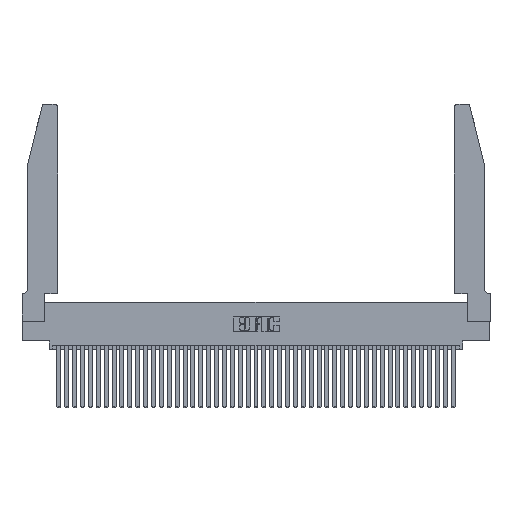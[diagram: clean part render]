
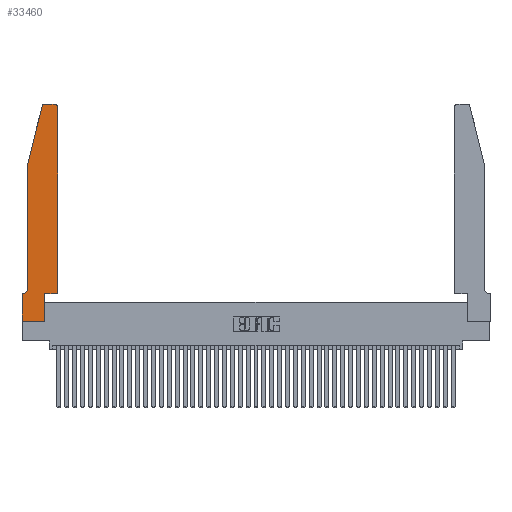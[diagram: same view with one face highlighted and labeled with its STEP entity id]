
A CAD part, top view. The second image highlights one B-rep face of the part: STEP entity #33460.
In plain terms, the highlighted planar face has unit normal (0, 0, 1).
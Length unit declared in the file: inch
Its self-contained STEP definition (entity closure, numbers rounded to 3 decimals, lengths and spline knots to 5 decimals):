
#149 = VECTOR ( 'NONE', #41170, 39.37008 ) ;
#591 = ORIENTED_EDGE ( 'NONE', *, *, #41050, .T. ) ;
#843 = CARTESIAN_POINT ( 'NONE',  ( 0.25487, 2.72718, 0.37 ) ) ;
#1195 = VECTOR ( 'NONE', #23266, 39.37008 ) ;
#1265 = LINE ( 'NONE', #6228, #8586 ) ;
#1380 = DIRECTION ( 'NONE',  ( -1., 0., 0. ) ) ;
#2826 = CARTESIAN_POINT ( 'NONE',  ( 0.0755, 0.35, 0.37 ) ) ;
#3348 = ORIENTED_EDGE ( 'NONE', *, *, #5975, .T. ) ;
#4459 = CARTESIAN_POINT ( 'NONE',  ( 0.2865, 0.35, 0.37 ) ) ;
#5761 = VERTEX_POINT ( 'NONE', #24829 ) ;
#5888 = ORIENTED_EDGE ( 'NONE', *, *, #37922, .T. ) ;
#5975 = EDGE_CURVE ( 'NONE', #10247, #7414, #9062, .T. ) ;
#6228 = CARTESIAN_POINT ( 'NONE',  ( 0., 0., 0.37 ) ) ;
#6584 = VECTOR ( 'NONE', #27744, 39.37008 ) ;
#6618 = VECTOR ( 'NONE', #22901, 39.37008 ) ;
#7010 = ORIENTED_EDGE ( 'NONE', *, *, #17214, .T. ) ;
#7385 = CARTESIAN_POINT ( 'NONE',  ( 0.284, 2.72, 0.37 ) ) ;
#7414 = VERTEX_POINT ( 'NONE', #34551 ) ;
#7542 = EDGE_CURVE ( 'NONE', #10661, #35341, #28443, .T. ) ;
#7826 = DIRECTION ( 'NONE',  ( 1., 0., 0. ) ) ;
#7898 = CARTESIAN_POINT ( 'NONE',  ( 0.4505, 0.35, 0.37 ) ) ;
#8586 = VECTOR ( 'NONE', #12844, 39.37008 ) ;
#8888 = VECTOR ( 'NONE', #24310, 39.37008 ) ;
#8977 = VECTOR ( 'NONE', #29935, 39.37008 ) ;
#9014 = VERTEX_POINT ( 'NONE', #22245 ) ;
#9062 = LINE ( 'NONE', #2826, #1195 ) ;
#9153 = CIRCLE ( 'NONE', #35508, 0.03 ) ;
#9172 = CARTESIAN_POINT ( 'NONE',  ( 0.4205, 2.75, 0.37 ) ) ;
#9303 = ORIENTED_EDGE ( 'NONE', *, *, #29310, .T. ) ;
#9967 = AXIS2_PLACEMENT_3D ( 'NONE', #7385, #27265, #30627 ) ;
#10138 = LINE ( 'NONE', #4459, #149 ) ;
#10247 = VERTEX_POINT ( 'NONE', #21009 ) ;
#10661 = VERTEX_POINT ( 'NONE', #9172 ) ;
#10894 = ORIENTED_EDGE ( 'NONE', *, *, #7542, .T. ) ;
#10961 = CARTESIAN_POINT ( 'NONE',  ( 0.0755, 2., 0.37 ) ) ;
#11203 = PLANE ( 'NONE',  #42043 ) ;
#11349 = CARTESIAN_POINT ( 'NONE',  ( 0., 0.35, 0.37 ) ) ;
#12844 = DIRECTION ( 'NONE',  ( 0., -1., 0. ) ) ;
#14658 = DIRECTION ( 'NONE',  ( 0., 0., -1. ) ) ;
#16202 = DIRECTION ( 'NONE',  ( 0., 0., 1. ) ) ;
#16878 = LINE ( 'NONE', #7898, #19493 ) ;
#17214 = EDGE_CURVE ( 'NONE', #35341, #30072, #18837, .T. ) ;
#17761 = CARTESIAN_POINT ( 'NONE',  ( 0.0755, 2., 0.37 ) ) ;
#17921 = LINE ( 'NONE', #24764, #8977 ) ;
#18352 = EDGE_CURVE ( 'NONE', #5761, #26841, #16878, .T. ) ;
#18398 = EDGE_CURVE ( 'NONE', #26841, #34080, #17921, .T. ) ;
#18837 = CIRCLE ( 'NONE', #9967, 0.03 ) ;
#19493 = VECTOR ( 'NONE', #28366, 39.37008 ) ;
#20409 = CARTESIAN_POINT ( 'NONE',  ( 0.2605, 2.75, 0.37 ) ) ;
#21009 = CARTESIAN_POINT ( 'NONE',  ( 0.0055, 0.35, 0.37 ) ) ;
#21439 = VERTEX_POINT ( 'NONE', #17761 ) ;
#21795 = CARTESIAN_POINT ( 'NONE',  ( 0.4505, 2.72, 0.37 ) ) ;
#22245 = CARTESIAN_POINT ( 'NONE',  ( 0.2865, 0., 0.37 ) ) ;
#22258 = CARTESIAN_POINT ( 'NONE',  ( 0.0755, 0.42, 0.37 ) ) ;
#22901 = DIRECTION ( 'NONE',  ( 0., -1., 0. ) ) ;
#23266 = DIRECTION ( 'NONE',  ( -1., 0., 0. ) ) ;
#23554 = VERTEX_POINT ( 'NONE', #22258 ) ;
#24310 = DIRECTION ( 'NONE',  ( 1., 0., 0. ) ) ;
#24764 = CARTESIAN_POINT ( 'NONE',  ( 0.4505, 0.35, 0.37 ) ) ;
#24829 = CARTESIAN_POINT ( 'NONE',  ( 0.2865, 0.35, 0.37 ) ) ;
#24857 = CARTESIAN_POINT ( 'NONE',  ( 0., 0., 0.37 ) ) ;
#25534 = ORIENTED_EDGE ( 'NONE', *, *, #18352, .T. ) ;
#25536 = ORIENTED_EDGE ( 'NONE', *, *, #37291, .T. ) ;
#26841 = VERTEX_POINT ( 'NONE', #43111 ) ;
#27265 = DIRECTION ( 'NONE',  ( 0., 0., 1. ) ) ;
#27547 = EDGE_CURVE ( 'NONE', #21439, #23554, #36650, .T. ) ;
#27744 = DIRECTION ( 'NONE',  ( -0.239, -0.971, 0. ) ) ;
#28271 = LINE ( 'NONE', #10961, #6584 ) ;
#28366 = DIRECTION ( 'NONE',  ( 1., 0., 0. ) ) ;
#28381 = ORIENTED_EDGE ( 'NONE', *, *, #37279, .T. ) ;
#28443 = LINE ( 'NONE', #20409, #42631 ) ;
#29310 = EDGE_CURVE ( 'NONE', #34080, #10661, #9153, .T. ) ;
#29935 = DIRECTION ( 'NONE',  ( 0., 1., 0. ) ) ;
#30072 = VERTEX_POINT ( 'NONE', #843 ) ;
#30408 = EDGE_LOOP ( 'NONE', ( #10894, #7010, #25536, #35994, #28381, #3348, #40941, #5888, #591, #25534, #38029, #9303 ) ) ;
#30627 = DIRECTION ( 'NONE',  ( 1., 0., 0. ) ) ;
#32799 = CARTESIAN_POINT ( 'NONE',  ( 0.4205, 2.72, 0.37 ) ) ;
#33460 = ADVANCED_FACE ( 'NONE', ( #33469 ), #11203, .T. ) ;
#33469 = FACE_OUTER_BOUND ( 'NONE', #30408, .T. ) ;
#34080 = VERTEX_POINT ( 'NONE', #21795 ) ;
#34312 = CARTESIAN_POINT ( 'NONE',  ( 0., 0., 0.37 ) ) ;
#34551 = CARTESIAN_POINT ( 'NONE',  ( 0., 0.35, 0.37 ) ) ;
#34752 = DIRECTION ( 'NONE',  ( 0., 0., 1. ) ) ;
#35109 = AXIS2_PLACEMENT_3D ( 'NONE', #41700, #14658, #37895 ) ;
#35142 = CARTESIAN_POINT ( 'NONE',  ( 0.0755, 2., 0.37 ) ) ;
#35341 = VERTEX_POINT ( 'NONE', #37178 ) ;
#35508 = AXIS2_PLACEMENT_3D ( 'NONE', #32799, #16202, #39472 ) ;
#35812 = EDGE_CURVE ( 'NONE', #7414, #36731, #1265, .T. ) ;
#35994 = ORIENTED_EDGE ( 'NONE', *, *, #27547, .T. ) ;
#36284 = LINE ( 'NONE', #34312, #8888 ) ;
#36650 = LINE ( 'NONE', #35142, #6618 ) ;
#36731 = VERTEX_POINT ( 'NONE', #24857 ) ;
#37178 = CARTESIAN_POINT ( 'NONE',  ( 0.284, 2.75, 0.37 ) ) ;
#37279 = EDGE_CURVE ( 'NONE', #23554, #10247, #40167, .T. ) ;
#37291 = EDGE_CURVE ( 'NONE', #30072, #21439, #28271, .T. ) ;
#37895 = DIRECTION ( 'NONE',  ( -1., 0., 0. ) ) ;
#37922 = EDGE_CURVE ( 'NONE', #36731, #9014, #36284, .T. ) ;
#38029 = ORIENTED_EDGE ( 'NONE', *, *, #18398, .T. ) ;
#39472 = DIRECTION ( 'NONE',  ( 1., 0., 0. ) ) ;
#40167 = CIRCLE ( 'NONE', #35109, 0.07 ) ;
#40941 = ORIENTED_EDGE ( 'NONE', *, *, #35812, .T. ) ;
#41050 = EDGE_CURVE ( 'NONE', #9014, #5761, #10138, .T. ) ;
#41170 = DIRECTION ( 'NONE',  ( 0., 1., 0. ) ) ;
#41700 = CARTESIAN_POINT ( 'NONE',  ( 0.0055, 0.42, 0.37 ) ) ;
#42043 = AXIS2_PLACEMENT_3D ( 'NONE', #11349, #34752, #7826 ) ;
#42631 = VECTOR ( 'NONE', #1380, 39.37008 ) ;
#43111 = CARTESIAN_POINT ( 'NONE',  ( 0.4505, 0.35, 0.37 ) ) ;
